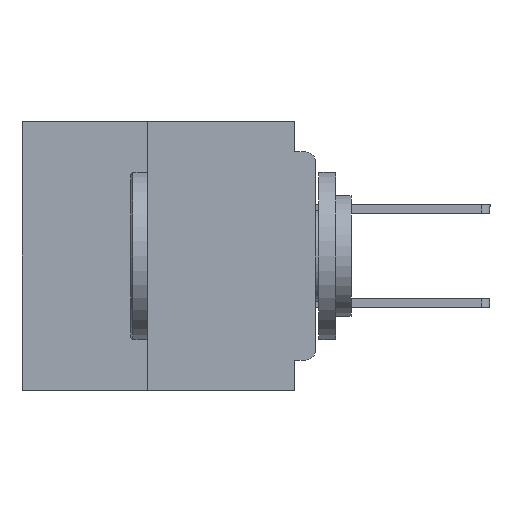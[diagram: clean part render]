
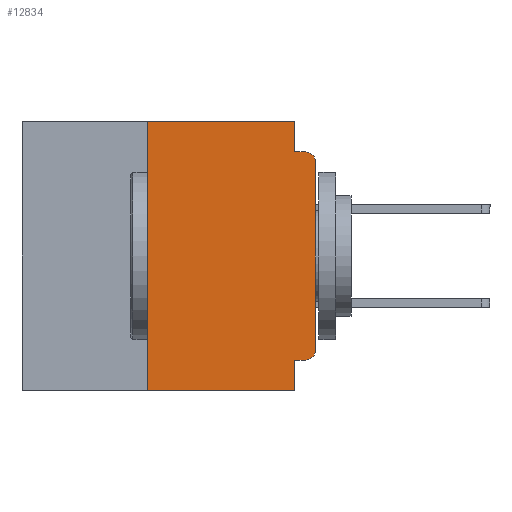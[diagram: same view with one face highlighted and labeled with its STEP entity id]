
A CAD part, left-side view. The second image highlights one B-rep face of the part: STEP entity #12834.
In plain terms, the highlighted planar face has unit normal (-1, 0, 0).
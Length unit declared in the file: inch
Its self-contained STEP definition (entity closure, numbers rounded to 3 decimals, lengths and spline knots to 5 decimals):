
#294 = VERTEX_POINT ( 'NONE', #26857 ) ;
#715 = CARTESIAN_POINT ( 'NONE',  ( 0., 0.031, 0. ) ) ;
#843 = LINE ( 'NONE', #6168, #35314 ) ;
#2115 = VECTOR ( 'NONE', #24054, 39.37008 ) ;
#2276 = VERTEX_POINT ( 'NONE', #33029 ) ;
#2578 = EDGE_CURVE ( 'NONE', #32771, #16864, #19938, .T. ) ;
#3061 = VERTEX_POINT ( 'NONE', #11213 ) ;
#3460 = ORIENTED_EDGE ( 'NONE', *, *, #7162, .F. ) ;
#4945 = AXIS2_PLACEMENT_3D ( 'NONE', #35883, #16057, #39236 ) ;
#4962 = VECTOR ( 'NONE', #13972, 39.37008 ) ;
#5079 = DIRECTION ( 'NONE',  ( 1., 0., 0. ) ) ;
#5081 = EDGE_CURVE ( 'NONE', #16864, #30383, #24990, .T. ) ;
#6168 = CARTESIAN_POINT ( 'NONE',  ( 0., 0.031, -0.4 ) ) ;
#6911 = CARTESIAN_POINT ( 'NONE',  ( 0., 0.25, 0. ) ) ;
#7162 = EDGE_CURVE ( 'NONE', #2276, #3061, #22200, .T. ) ;
#7183 = CARTESIAN_POINT ( 'NONE',  ( 0., 0., -0.06 ) ) ;
#8301 = VECTOR ( 'NONE', #24017, 39.37008 ) ;
#10724 = VECTOR ( 'NONE', #21282, 39.37008 ) ;
#11213 = CARTESIAN_POINT ( 'NONE',  ( 0., 0.015, -0.045 ) ) ;
#11796 = LINE ( 'NONE', #37815, #10724 ) ;
#12733 = FACE_OUTER_BOUND ( 'NONE', #36247, .T. ) ;
#12834 = ADVANCED_FACE ( 'NONE', ( #12733 ), #41600, .F. ) ;
#12905 = CARTESIAN_POINT ( 'NONE',  ( 0., 0.25, -0.4 ) ) ;
#13020 = ORIENTED_EDGE ( 'NONE', *, *, #22266, .F. ) ;
#13072 = CARTESIAN_POINT ( 'NONE',  ( 0., 0., -0.045 ) ) ;
#13492 = DIRECTION ( 'NONE',  ( 0., 0., 1. ) ) ;
#13789 = CARTESIAN_POINT ( 'NONE',  ( 0., 0.031, -0.355 ) ) ;
#13931 = LINE ( 'NONE', #33799, #4962 ) ;
#13972 = DIRECTION ( 'NONE',  ( 0., -1., 0. ) ) ;
#14345 = DIRECTION ( 'NONE',  ( -1., 0., 0. ) ) ;
#15457 = VERTEX_POINT ( 'NONE', #26051 ) ;
#16057 = DIRECTION ( 'NONE',  ( -1., 0., 0. ) ) ;
#16413 = DIRECTION ( 'NONE',  ( 0., -1., 0. ) ) ;
#16864 = VERTEX_POINT ( 'NONE', #6911 ) ;
#17670 = ORIENTED_EDGE ( 'NONE', *, *, #2578, .F. ) ;
#17866 = EDGE_CURVE ( 'NONE', #15457, #25220, #31704, .T. ) ;
#19132 = CARTESIAN_POINT ( 'NONE',  ( 0., 0.031, 0. ) ) ;
#19176 = ORIENTED_EDGE ( 'NONE', *, *, #39550, .T. ) ;
#19909 = EDGE_CURVE ( 'NONE', #30383, #2276, #25932, .T. ) ;
#19938 = LINE ( 'NONE', #23256, #2115 ) ;
#20690 = AXIS2_PLACEMENT_3D ( 'NONE', #25055, #5079, #28373 ) ;
#20813 = EDGE_CURVE ( 'NONE', #40352, #15457, #34694, .T. ) ;
#21282 = DIRECTION ( 'NONE',  ( 0., 1., 0. ) ) ;
#22200 = LINE ( 'NONE', #13072, #38813 ) ;
#22266 = EDGE_CURVE ( 'NONE', #40352, #35853, #11796, .T. ) ;
#23256 = CARTESIAN_POINT ( 'NONE',  ( 0., 0.25, -0.4 ) ) ;
#23898 = ORIENTED_EDGE ( 'NONE', *, *, #20813, .T. ) ;
#23921 = VECTOR ( 'NONE', #13492, 39.37008 ) ;
#24017 = DIRECTION ( 'NONE',  ( 0., 0., -1. ) ) ;
#24054 = DIRECTION ( 'NONE',  ( 0., 0., 1. ) ) ;
#24668 = CARTESIAN_POINT ( 'NONE',  ( 0., 0.015, -0.355 ) ) ;
#24990 = LINE ( 'NONE', #29651, #32759 ) ;
#25055 = CARTESIAN_POINT ( 'NONE',  ( 0., 0.437, 0. ) ) ;
#25220 = VERTEX_POINT ( 'NONE', #7183 ) ;
#25932 = LINE ( 'NONE', #715, #8301 ) ;
#26051 = CARTESIAN_POINT ( 'NONE',  ( 0., 0., -0.34 ) ) ;
#26433 = EDGE_CURVE ( 'NONE', #32771, #294, #13931, .T. ) ;
#26857 = CARTESIAN_POINT ( 'NONE',  ( 0., 0.031, -0.4 ) ) ;
#27840 = CIRCLE ( 'NONE', #30948, 0.015 ) ;
#28373 = DIRECTION ( 'NONE',  ( 0., 0., -1. ) ) ;
#29573 = ORIENTED_EDGE ( 'NONE', *, *, #43083, .F. ) ;
#29651 = CARTESIAN_POINT ( 'NONE',  ( 0., 0.437, 0. ) ) ;
#30068 = ORIENTED_EDGE ( 'NONE', *, *, #19909, .F. ) ;
#30339 = DIRECTION ( 'NONE',  ( 0., -1., 0. ) ) ;
#30383 = VERTEX_POINT ( 'NONE', #19132 ) ;
#30948 = AXIS2_PLACEMENT_3D ( 'NONE', #34156, #14345, #37476 ) ;
#31123 = ORIENTED_EDGE ( 'NONE', *, *, #5081, .F. ) ;
#31704 = LINE ( 'NONE', #33324, #23921 ) ;
#32759 = VECTOR ( 'NONE', #30339, 39.37008 ) ;
#32771 = VERTEX_POINT ( 'NONE', #12905 ) ;
#33029 = CARTESIAN_POINT ( 'NONE',  ( 0., 0.031, -0.045 ) ) ;
#33324 = CARTESIAN_POINT ( 'NONE',  ( 0., 0., 0. ) ) ;
#33799 = CARTESIAN_POINT ( 'NONE',  ( 0., 0.437, -0.4 ) ) ;
#34156 = CARTESIAN_POINT ( 'NONE',  ( 0., 0.015, -0.06 ) ) ;
#34694 = CIRCLE ( 'NONE', #4945, 0.015 ) ;
#35285 = ORIENTED_EDGE ( 'NONE', *, *, #26433, .T. ) ;
#35314 = VECTOR ( 'NONE', #36123, 39.37008 ) ;
#35853 = VERTEX_POINT ( 'NONE', #13789 ) ;
#35883 = CARTESIAN_POINT ( 'NONE',  ( 0., 0.015, -0.34 ) ) ;
#36123 = DIRECTION ( 'NONE',  ( 0., 0., -1. ) ) ;
#36247 = EDGE_LOOP ( 'NONE', ( #40753, #19176, #3460, #30068, #31123, #17670, #35285, #29573, #13020, #23898 ) ) ;
#37476 = DIRECTION ( 'NONE',  ( 0., 0., -1. ) ) ;
#37815 = CARTESIAN_POINT ( 'NONE',  ( 0., 0., -0.355 ) ) ;
#38813 = VECTOR ( 'NONE', #16413, 39.37008 ) ;
#39236 = DIRECTION ( 'NONE',  ( 0., 0., -1. ) ) ;
#39550 = EDGE_CURVE ( 'NONE', #25220, #3061, #27840, .T. ) ;
#40352 = VERTEX_POINT ( 'NONE', #24668 ) ;
#40753 = ORIENTED_EDGE ( 'NONE', *, *, #17866, .T. ) ;
#41600 = PLANE ( 'NONE',  #20690 ) ;
#43083 = EDGE_CURVE ( 'NONE', #35853, #294, #843, .T. ) ;
